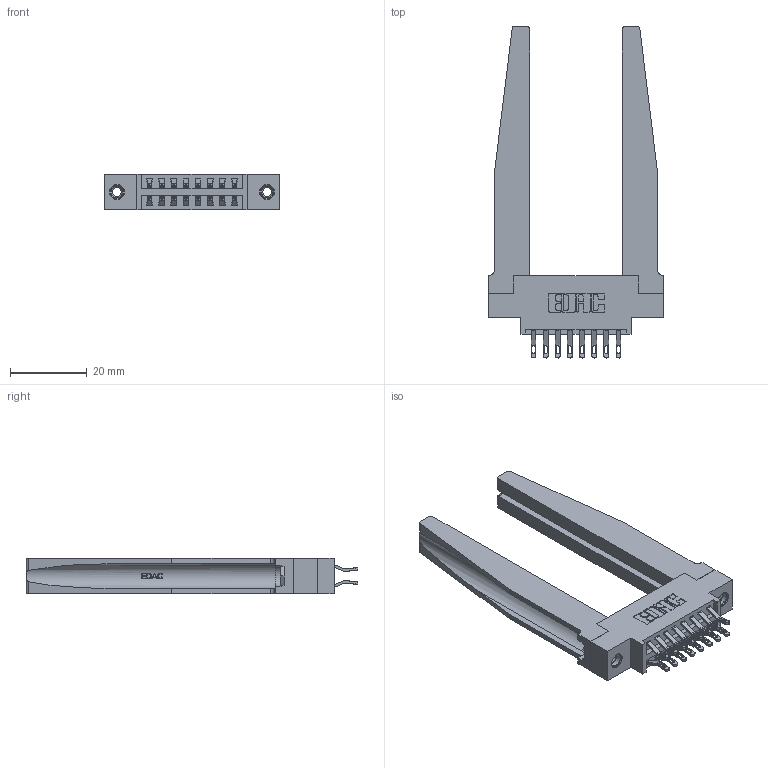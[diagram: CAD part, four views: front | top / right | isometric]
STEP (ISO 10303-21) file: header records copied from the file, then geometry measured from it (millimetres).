
FILE_DESCRIPTION (( 'STEP AP203' ), '1' );
FILE_NAME ('346-016-555-878.STEP', '2022-05-18T16:12:18', ( '' ), ( '' ), 'SwSTEP 2.0', 'SolidWorks 2020', '' );
FILE_SCHEMA (( 'CONFIG_CONTROL_DESIGN' ));
Length unit declared in the file: inch
Products named in the file (5): 345-250-001_345-250-001-102; 345-292-001_555 Tail; 346-016-555-878; 346-220-078_345-220-078; 346 Part_0.170 Offset - 0.156 Dia-TH
Assembly tree (21 placements, depth 2):
  346-016-555-878
    346 Part_0.170 Offset - 0.156 Dia-TH
    345-292-001_555 Tail  x16
    346-220-078_345-220-078  x2
    345-250-001_345-250-001-102  x2
Bounding box: 45.97 x 86.74 x 9.4 mm (x, y, z)
Volume: 11001.5 mm3; surface area: 12008.4 mm2
Topology: 21 solids, 21 shells, 1302 faces, 3913 edges, 2598 vertices
Faces by surface type: plane 764, cylinder 486, bspline 36, cone 12, torus 4
Entity records: 15420 total; most frequent: CARTESIAN_POINT 3567, ORIENTED_EDGE 2358, DIRECTION 2149, EDGE_CURVE 1179, VECTOR 901, LINE 901, VERTEX_POINT 780, AXIS2_PLACEMENT_3D 624
